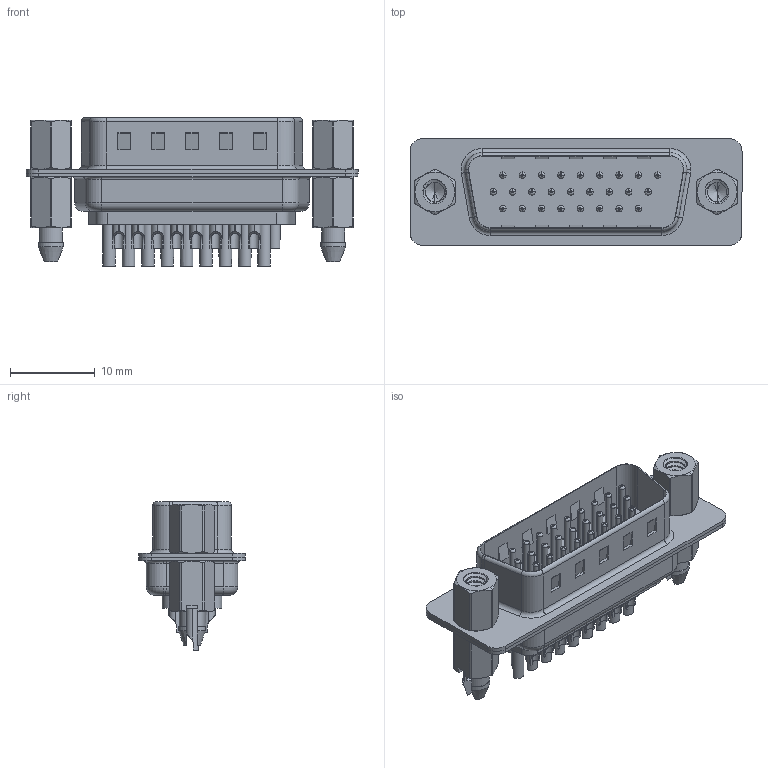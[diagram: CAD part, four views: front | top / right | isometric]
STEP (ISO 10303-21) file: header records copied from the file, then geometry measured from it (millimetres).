
FILE_DESCRIPTION (( 'STEP AP203' ), '1' );
FILE_NAME ('637-026-632-067.STEP', '2020-07-18T01:31:44', ( '' ), ( '' ), 'SwSTEP 2.0', 'SolidWorks 2020', '' );
FILE_SCHEMA (( 'CONFIG_CONTROL_DESIGN' ));
Length unit declared in the file: millimetre
Products named in the file (9): 637 Contact Row 3_32; 637 4-40 Threaded Boardlock_LP; 637 Shell Front_26 Contacts; 637 Shell Rear_26 Contacts; 637 Contact Row 2_32; 637 Housing_26 Contacts; 637 Contact Row 1_32; 637 4-40 Hex Standoff; 637-026-632-067
Assembly tree (33 placements, depth 2):
  637-026-632-067
    637 Housing_26 Contacts
    637 Shell Front_26 Contacts
    637 Shell Rear_26 Contacts
    637 Contact Row 1_32  x9
    637 Contact Row 2_32  x9
    637 Contact Row 3_32  x8
    637 4-40 Hex Standoff  x2
    637 4-40 Threaded Boardlock_LP  x2
Bounding box: 39.2 x 12.6 x 17.55 mm (x, y, z)
Volume: 2180.1 mm3; surface area: 7695.3 mm2
Topology: 33 solids, 33 shells, 2204 faces, 5701 edges, 3624 vertices
Faces by surface type: cylinder 991, torus 596, plane 557, cone 42, bspline 18
Entity records: 29455 total; most frequent: CARTESIAN_POINT 8508, DIRECTION 4270, ORIENTED_EDGE 3940, EDGE_CURVE 1970, AXIS2_PLACEMENT_3D 1707, VERTEX_POINT 1265, EDGE_LOOP 931, CIRCLE 897
